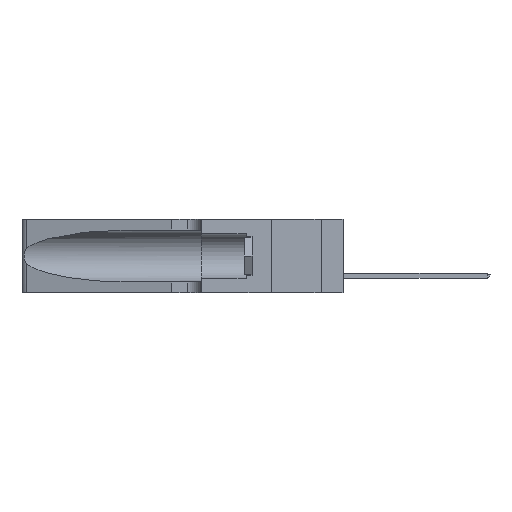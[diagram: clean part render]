
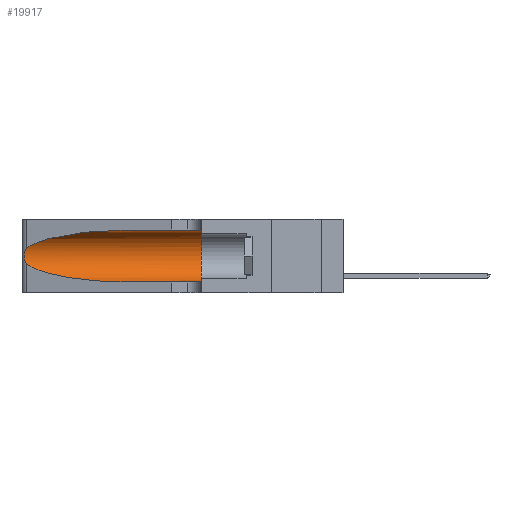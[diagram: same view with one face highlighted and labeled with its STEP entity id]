
A CAD part, left-side view. The second image highlights one B-rep face of the part: STEP entity #19917.
In plain terms, the highlighted cylindrical face has radius 3.308 mm (diameter 6.617 mm), a partial arc.
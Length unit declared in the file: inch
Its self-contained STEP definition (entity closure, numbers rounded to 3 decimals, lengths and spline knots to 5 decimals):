
#291 = CARTESIAN_POINT ( 'NONE',  ( 0.25487, 1.22718, 0.14631 ) ) ;
#857 = CARTESIAN_POINT ( 'NONE',  ( 0.25787, 1.23484, 0.2124 ) ) ;
#1280 = ORIENTED_EDGE ( 'NONE', *, *, #8441, .T. ) ;
#1906 = LINE ( 'NONE', #14068, #15983 ) ;
#2033 = VERTEX_POINT ( 'NONE', #21816 ) ;
#2824 = CARTESIAN_POINT ( 'NONE',  ( 0.26075, 1.23896, 0.19203 ) ) ;
#2847 = CYLINDRICAL_SURFACE ( 'NONE', #14635, 0.13025 ) ;
#3049 = B_SPLINE_CURVE_WITH_KNOTS ( 'NONE', 3,
 ( #8983, #21633, #25547, #857, #7037, #14850, #2824, #6866, #10911, #13451, #15486, #24907, #3636, #12732 ),
 .UNSPECIFIED., .F., .F.,
 ( 4, 2, 2, 2, 2, 2, 4 ),
 ( 0., 0.00027, 0.00053, 0.00107, 0.0016, 0.00187, 0.00214 ),
 .UNSPECIFIED. ) ;
#3601 = CARTESIAN_POINT ( 'NONE',  ( 0.1305, 0.35, 0.31525 ) ) ;
#3636 = CARTESIAN_POINT ( 'NONE',  ( 0.25555, 1.22993, 0.14849 ) ) ;
#4530 = CARTESIAN_POINT ( 'NONE',  ( 0.2373, 1.15595, 0.28018 ) ) ;
#4818 = CARTESIAN_POINT ( 'NONE',  ( 0.25487, 1.22718, 0.14631 ) ) ;
#4957 = LINE ( 'NONE', #14914, #10632 ) ;
#6290 = ORIENTED_EDGE ( 'NONE', *, *, #15653, .T. ) ;
#6318 = DIRECTION ( 'NONE',  ( 0., 0., 1. ) ) ;
#6556 = CARTESIAN_POINT ( 'NONE',  ( 0.25487, 1.22718, 0.22369 ) ) ;
#6866 = CARTESIAN_POINT ( 'NONE',  ( 0.26075, 1.23896, 0.178 ) ) ;
#7037 = CARTESIAN_POINT ( 'NONE',  ( 0.25854, 1.2359, 0.20912 ) ) ;
#7880 = DIRECTION ( 'NONE',  ( 0., -1., 0. ) ) ;
#8441 = EDGE_CURVE ( 'NONE', #13047, #2033, #14299, .T. ) ;
#8846 = CARTESIAN_POINT ( 'NONE',  ( 0.1305, 0.72297, 0.31525 ) ) ;
#8983 = CARTESIAN_POINT ( 'NONE',  ( 0.25487, 1.22718, 0.22369 ) ) ;
#9229 = DIRECTION ( 'NONE',  ( 0., -1., 0. ) ) ;
#9688 =( BOUNDED_CURVE ( )  B_SPLINE_CURVE ( 3, ( #291, #24231, #12256, #14433 ),
 .UNSPECIFIED., .F., .F. ) 
 B_SPLINE_CURVE_WITH_KNOTS ( ( 4, 4 ),
 ( 3.44316, 4.71239 ),
 .UNSPECIFIED. ) 
 CURVE ( )  GEOMETRIC_REPRESENTATION_ITEM ( )  RATIONAL_B_SPLINE_CURVE ( ( 1., 0.87, 0.87, 1. ) ) 
 REPRESENTATION_ITEM ( '' )  );
#9901 = VERTEX_POINT ( 'NONE', #18898 ) ;
#9909 = EDGE_CURVE ( 'NONE', #2033, #20649, #3049, .T. ) ;
#10003 = ORIENTED_EDGE ( 'NONE', *, *, #10209, .F. ) ;
#10209 = EDGE_CURVE ( 'NONE', #13271, #21416, #17313, .T. ) ;
#10632 = VECTOR ( 'NONE', #9229, 39.37008 ) ;
#10911 = CARTESIAN_POINT ( 'NONE',  ( 0.26017, 1.23833, 0.17102 ) ) ;
#11738 = AXIS2_PLACEMENT_3D ( 'NONE', #24717, #12703, #6318 ) ;
#12207 = EDGE_CURVE ( 'NONE', #9901, #21416, #4957, .T. ) ;
#12256 = CARTESIAN_POINT ( 'NONE',  ( 0.18966, 0.96281, 0.05475 ) ) ;
#12703 = DIRECTION ( 'NONE',  ( 0., 1., 0. ) ) ;
#12732 = CARTESIAN_POINT ( 'NONE',  ( 0.25487, 1.22718, 0.14631 ) ) ;
#13047 = VERTEX_POINT ( 'NONE', #21635 ) ;
#13271 = VERTEX_POINT ( 'NONE', #3601 ) ;
#13311 = CARTESIAN_POINT ( 'NONE',  ( 0.1305, 1.61858, 0.185 ) ) ;
#13451 = CARTESIAN_POINT ( 'NONE',  ( 0.25856, 1.23593, 0.16098 ) ) ;
#14068 = CARTESIAN_POINT ( 'NONE',  ( 0.1305, 1.61858, 0.31525 ) ) ;
#14299 =( BOUNDED_CURVE ( )  B_SPLINE_CURVE ( 3, ( #8846, #24512, #4530, #6556 ),
 .UNSPECIFIED., .F., .F. ) 
 B_SPLINE_CURVE_WITH_KNOTS ( ( 4, 4 ),
 ( 1.5708, 2.84003 ),
 .UNSPECIFIED. ) 
 CURVE ( )  GEOMETRIC_REPRESENTATION_ITEM ( )  RATIONAL_B_SPLINE_CURVE ( ( 1., 0.87, 0.87, 1. ) ) 
 REPRESENTATION_ITEM ( '' )  );
#14433 = CARTESIAN_POINT ( 'NONE',  ( 0.1305, 0.72297, 0.05475 ) ) ;
#14635 = AXIS2_PLACEMENT_3D ( 'NONE', #13311, #15165, #15347 ) ;
#14831 = CARTESIAN_POINT ( 'NONE',  ( 0.1305, 0.35, 0.05475 ) ) ;
#14850 = CARTESIAN_POINT ( 'NONE',  ( 0.26018, 1.23835, 0.19895 ) ) ;
#14914 = CARTESIAN_POINT ( 'NONE',  ( 0.1305, 1.61858, 0.05475 ) ) ;
#15165 = DIRECTION ( 'NONE',  ( 0., -1., 0. ) ) ;
#15347 = DIRECTION ( 'NONE',  ( 0., 0., -1. ) ) ;
#15486 = CARTESIAN_POINT ( 'NONE',  ( 0.25789, 1.23486, 0.15765 ) ) ;
#15653 = EDGE_CURVE ( 'NONE', #20649, #9901, #9688, .T. ) ;
#15887 = ORIENTED_EDGE ( 'NONE', *, *, #9909, .T. ) ;
#15983 = VECTOR ( 'NONE', #7880, 39.37008 ) ;
#17313 = CIRCLE ( 'NONE', #11738, 0.13025 ) ;
#17990 = EDGE_LOOP ( 'NONE', ( #1280, #15887, #6290, #20267, #10003, #24917 ) ) ;
#18898 = CARTESIAN_POINT ( 'NONE',  ( 0.1305, 0.72297, 0.05475 ) ) ;
#19917 = ADVANCED_FACE ( 'NONE', ( #25788 ), #2847, .F. ) ;
#20267 = ORIENTED_EDGE ( 'NONE', *, *, #12207, .T. ) ;
#20649 = VERTEX_POINT ( 'NONE', #4818 ) ;
#21416 = VERTEX_POINT ( 'NONE', #14831 ) ;
#21633 = CARTESIAN_POINT ( 'NONE',  ( 0.25555, 1.22994, 0.2215 ) ) ;
#21635 = CARTESIAN_POINT ( 'NONE',  ( 0.1305, 0.72297, 0.31525 ) ) ;
#21816 = CARTESIAN_POINT ( 'NONE',  ( 0.25487, 1.22718, 0.22369 ) ) ;
#22374 = EDGE_CURVE ( 'NONE', #13047, #13271, #1906, .T. ) ;
#24231 = CARTESIAN_POINT ( 'NONE',  ( 0.2373, 1.15595, 0.08982 ) ) ;
#24512 = CARTESIAN_POINT ( 'NONE',  ( 0.18966, 0.96281, 0.31525 ) ) ;
#24717 = CARTESIAN_POINT ( 'NONE',  ( 0.1305, 0.35, 0.185 ) ) ;
#24907 = CARTESIAN_POINT ( 'NONE',  ( 0.25639, 1.23186, 0.15144 ) ) ;
#24917 = ORIENTED_EDGE ( 'NONE', *, *, #22374, .F. ) ;
#25547 = CARTESIAN_POINT ( 'NONE',  ( 0.25639, 1.23184, 0.21858 ) ) ;
#25788 = FACE_OUTER_BOUND ( 'NONE', #17990, .T. ) ;
